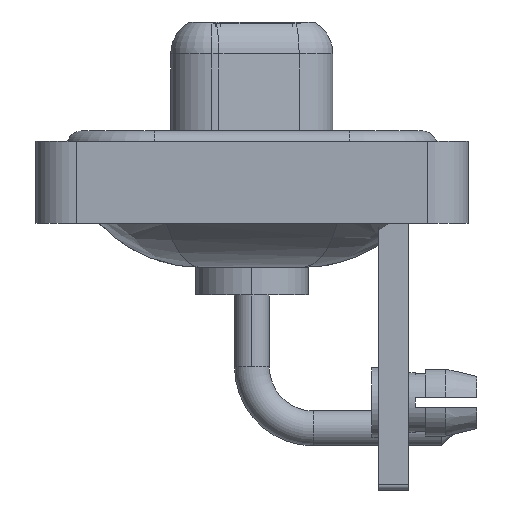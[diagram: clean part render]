
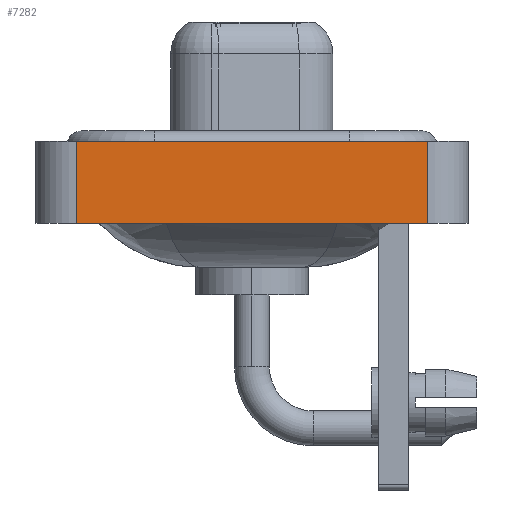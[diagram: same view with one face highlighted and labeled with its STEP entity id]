
A CAD part, left-side view. The second image highlights one B-rep face of the part: STEP entity #7282.
In plain terms, the highlighted planar face has unit normal (-1, 0, 0).
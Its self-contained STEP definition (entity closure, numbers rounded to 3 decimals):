
#669 = ORIENTED_EDGE ( 'NONE', *, *, #7138, .T. ) ;
#1857 = DIRECTION ( 'NONE',  ( 0., 0., 1. ) ) ;
#3939 = EDGE_CURVE ( 'NONE', #14812, #9118, #8381, .T. ) ;
#4219 = EDGE_CURVE ( 'NONE', #17878, #9118, #10497, .T. ) ;
#4275 = DIRECTION ( 'NONE',  ( 0., -1., 0. ) ) ;
#4538 = DIRECTION ( 'NONE',  ( 0., -1., 0. ) ) ;
#5042 = EDGE_CURVE ( 'NONE', #12874, #14812, #6679, .T. ) ;
#5779 = CARTESIAN_POINT ( 'NONE',  ( -7.35, -8.55, -3.6 ) ) ;
#6679 = LINE ( 'NONE', #13453, #10273 ) ;
#6920 = DIRECTION ( 'NONE',  ( 0., 0., 1. ) ) ;
#7138 = EDGE_CURVE ( 'NONE', #12874, #17878, #13265, .T. ) ;
#7282 = ADVANCED_FACE ( 'NONE', ( #18327 ), #17164, .T. ) ;
#7381 = CARTESIAN_POINT ( 'NONE',  ( -7.35, 8.55, -3.6 ) ) ;
#8381 = LINE ( 'NONE', #17389, #17589 ) ;
#8520 = CARTESIAN_POINT ( 'NONE',  ( -7.35, -8.55, 0.4 ) ) ;
#8539 = EDGE_LOOP ( 'NONE', ( #15893, #17721, #14105, #669 ) ) ;
#9055 = DIRECTION ( 'NONE',  ( 0., 0., 1. ) ) ;
#9118 = VERTEX_POINT ( 'NONE', #8520 ) ;
#9120 = CARTESIAN_POINT ( 'NONE',  ( -7.35, 8.55, 0.4 ) ) ;
#9793 = DIRECTION ( 'NONE',  ( -1., 0., 0. ) ) ;
#10273 = VECTOR ( 'NONE', #1857, 1000. ) ;
#10497 = LINE ( 'NONE', #16333, #12419 ) ;
#11946 = AXIS2_PLACEMENT_3D ( 'NONE', #12763, #9793, #6920 ) ;
#12419 = VECTOR ( 'NONE', #9055, 1000. ) ;
#12763 = CARTESIAN_POINT ( 'NONE',  ( -7.35, -8.55, -3.6 ) ) ;
#12874 = VERTEX_POINT ( 'NONE', #7381 ) ;
#13265 = LINE ( 'NONE', #5779, #15930 ) ;
#13453 = CARTESIAN_POINT ( 'NONE',  ( -7.35, 8.55, -3.6 ) ) ;
#13985 = CARTESIAN_POINT ( 'NONE',  ( -7.35, -8.55, -3.6 ) ) ;
#14105 = ORIENTED_EDGE ( 'NONE', *, *, #5042, .F. ) ;
#14812 = VERTEX_POINT ( 'NONE', #9120 ) ;
#15893 = ORIENTED_EDGE ( 'NONE', *, *, #4219, .T. ) ;
#15930 = VECTOR ( 'NONE', #4538, 1000. ) ;
#16333 = CARTESIAN_POINT ( 'NONE',  ( -7.35, -8.55, -3.6 ) ) ;
#17164 = PLANE ( 'NONE',  #11946 ) ;
#17389 = CARTESIAN_POINT ( 'NONE',  ( -7.35, -8.55, 0.4 ) ) ;
#17589 = VECTOR ( 'NONE', #4275, 1000. ) ;
#17721 = ORIENTED_EDGE ( 'NONE', *, *, #3939, .F. ) ;
#17878 = VERTEX_POINT ( 'NONE', #13985 ) ;
#18327 = FACE_OUTER_BOUND ( 'NONE', #8539, .T. ) ;
